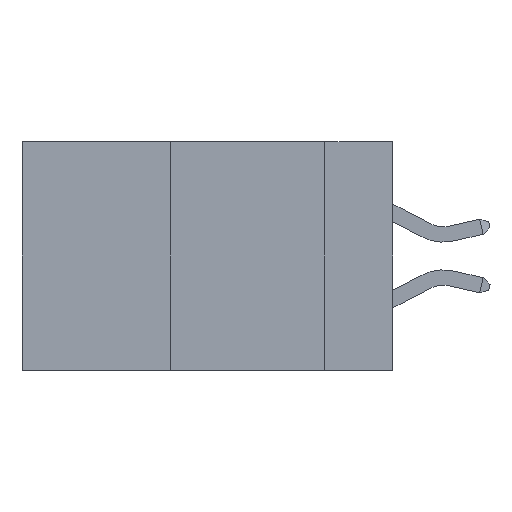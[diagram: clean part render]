
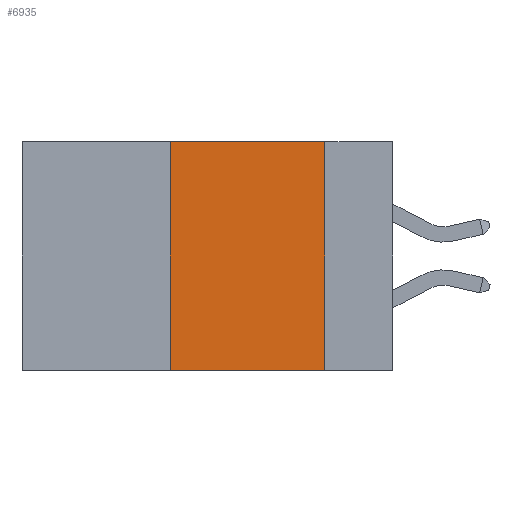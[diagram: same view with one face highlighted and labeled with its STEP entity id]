
A CAD part, left-side view. The second image highlights one B-rep face of the part: STEP entity #6935.
In plain terms, the highlighted planar face has unit normal (-1, 0, 0).
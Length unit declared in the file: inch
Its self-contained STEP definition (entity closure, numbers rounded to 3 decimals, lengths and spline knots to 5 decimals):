
#243 = LINE ( 'NONE', #506, #7221 ) ;
#258 = ORIENTED_EDGE ( 'NONE', *, *, #4075, .T. ) ;
#506 = CARTESIAN_POINT ( 'NONE',  ( 0., 0.6, -0.37 ) ) ;
#836 = AXIS2_PLACEMENT_3D ( 'NONE', #3868, #8324, #10020 ) ;
#1363 = LINE ( 'NONE', #5828, #3560 ) ;
#1381 = PLANE ( 'NONE',  #836 ) ;
#2365 = DIRECTION ( 'NONE',  ( 0., 0., -1. ) ) ;
#2421 = DIRECTION ( 'NONE',  ( 0., 0., 1. ) ) ;
#2941 = ORIENTED_EDGE ( 'NONE', *, *, #11102, .F. ) ;
#3468 = LINE ( 'NONE', #10195, #11030 ) ;
#3560 = VECTOR ( 'NONE', #5192, 39.37008 ) ;
#3868 = CARTESIAN_POINT ( 'NONE',  ( 0., 0.6, 0. ) ) ;
#4075 = EDGE_CURVE ( 'NONE', #8827, #5714, #243, .T. ) ;
#4107 = EDGE_CURVE ( 'NONE', #4781, #4248, #1363, .T. ) ;
#4248 = VERTEX_POINT ( 'NONE', #4387 ) ;
#4387 = CARTESIAN_POINT ( 'NONE',  ( 0., 0.11, 0. ) ) ;
#4472 = CARTESIAN_POINT ( 'NONE',  ( 0., 0.36, -0.37 ) ) ;
#4781 = VERTEX_POINT ( 'NONE', #9985 ) ;
#4963 = CARTESIAN_POINT ( 'NONE',  ( 0., 0.11, -0.37 ) ) ;
#5003 = DIRECTION ( 'NONE',  ( 0., -1., 0. ) ) ;
#5192 = DIRECTION ( 'NONE',  ( 0., -1., 0. ) ) ;
#5698 = ORIENTED_EDGE ( 'NONE', *, *, #8523, .F. ) ;
#5714 = VERTEX_POINT ( 'NONE', #4963 ) ;
#5828 = CARTESIAN_POINT ( 'NONE',  ( 0., 0.6, 0. ) ) ;
#5844 = CARTESIAN_POINT ( 'NONE',  ( 0., 0.36, 0. ) ) ;
#6935 = ADVANCED_FACE ( 'NONE', ( #7168 ), #1381, .F. ) ;
#7168 = FACE_OUTER_BOUND ( 'NONE', #7268, .T. ) ;
#7221 = VECTOR ( 'NONE', #5003, 39.37008 ) ;
#7268 = EDGE_LOOP ( 'NONE', ( #5698, #7854, #2941, #258 ) ) ;
#7526 = LINE ( 'NONE', #5844, #8894 ) ;
#7854 = ORIENTED_EDGE ( 'NONE', *, *, #4107, .F. ) ;
#8324 = DIRECTION ( 'NONE',  ( 1., 0., 0. ) ) ;
#8523 = EDGE_CURVE ( 'NONE', #4248, #5714, #3468, .T. ) ;
#8827 = VERTEX_POINT ( 'NONE', #4472 ) ;
#8894 = VECTOR ( 'NONE', #2421, 39.37008 ) ;
#9985 = CARTESIAN_POINT ( 'NONE',  ( 0., 0.36, 0. ) ) ;
#10020 = DIRECTION ( 'NONE',  ( 0., 0., -1. ) ) ;
#10195 = CARTESIAN_POINT ( 'NONE',  ( 0., 0.11, 0. ) ) ;
#11030 = VECTOR ( 'NONE', #2365, 39.37008 ) ;
#11102 = EDGE_CURVE ( 'NONE', #8827, #4781, #7526, .T. ) ;
